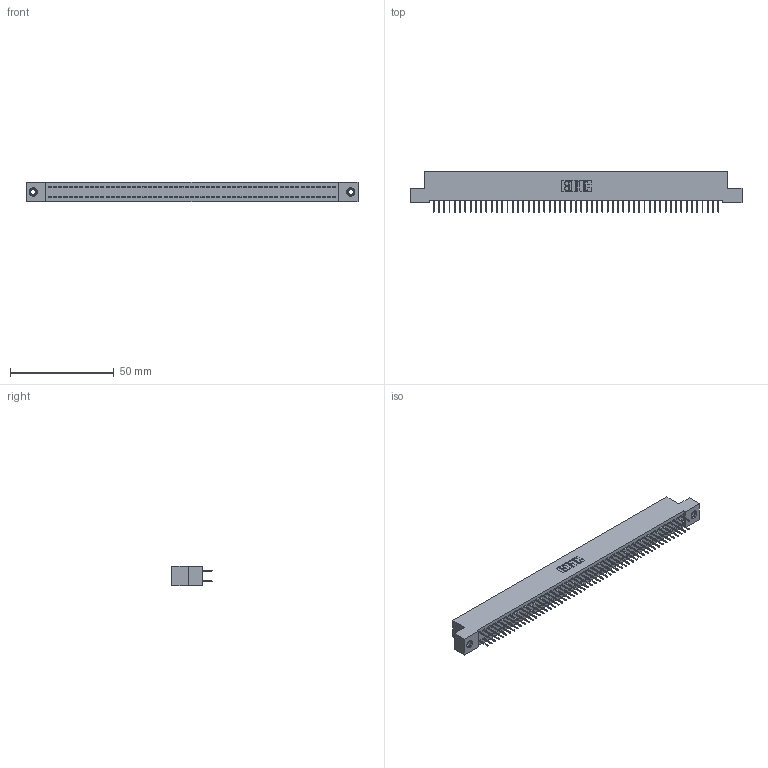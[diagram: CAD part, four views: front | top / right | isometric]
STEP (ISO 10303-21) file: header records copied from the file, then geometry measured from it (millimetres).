
FILE_DESCRIPTION (( 'STEP AP203' ), '1' );
FILE_NAME ('392-110-524-207.STEP', '2019-10-09T23:41:59', ( '' ), ( '' ), 'SwSTEP 2.0', 'SolidWorks 2016', '' );
FILE_SCHEMA (( 'CONFIG_CONTROL_DESIGN' ));
Length unit declared in the file: inch
Products named in the file (4): 345-250-001_345-250-005-103; 392-110-524-207; 342 Part_TI; 345-292-001_345-293-124
Assembly tree (113 placements, depth 2):
  392-110-524-207
    342 Part_TI
    345-292-001_345-293-124  x110
    345-250-001_345-250-005-103  x2
Bounding box: 160.02 x 19.69 x 9.4 mm (x, y, z)
Volume: 14260.2 mm3; surface area: 23125.1 mm2
Topology: 113 solids, 113 shells, 6330 faces, 17925 edges, 11502 vertices
Faces by surface type: plane 4718, cylinder 1596, cone 12, torus 4
Entity records: 34830 total; most frequent: CARTESIAN_POINT 5737, ORIENTED_EDGE 5666, DIRECTION 4911, EDGE_CURVE 2833, LINE 2689, VECTOR 2689, VERTEX_POINT 1880, AXIS2_PLACEMENT_3D 1111
